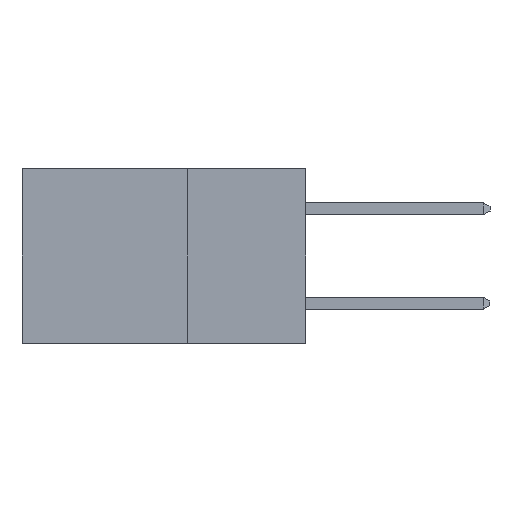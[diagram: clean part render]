
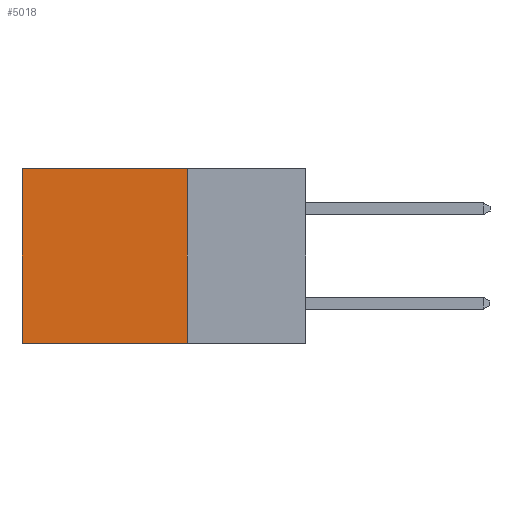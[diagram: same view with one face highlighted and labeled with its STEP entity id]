
A CAD part, left-side view. The second image highlights one B-rep face of the part: STEP entity #5018.
In plain terms, the highlighted planar face has unit normal (-1, 0, 0).
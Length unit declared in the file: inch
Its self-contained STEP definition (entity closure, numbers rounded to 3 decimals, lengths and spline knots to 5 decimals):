
#1595 = CARTESIAN_POINT ( 'NONE',  ( 0.298, 0.25, 0. ) ) ;
#2905 = LINE ( 'NONE', #28155, #13334 ) ;
#3591 = DIRECTION ( 'NONE',  ( 0., 0., -1. ) ) ;
#3656 = DIRECTION ( 'NONE',  ( 1., 0., 0. ) ) ;
#3760 = CARTESIAN_POINT ( 'NONE',  ( 0.298, 0.25, 0. ) ) ;
#3826 = CARTESIAN_POINT ( 'NONE',  ( 0.298, 0.25, -0.37 ) ) ;
#3869 = PLANE ( 'NONE',  #18601 ) ;
#3949 = VERTEX_POINT ( 'NONE', #1595 ) ;
#4423 = CARTESIAN_POINT ( 'NONE',  ( 0.298, 0.25, 0. ) ) ;
#4976 = ORIENTED_EDGE ( 'NONE', *, *, #10635, .T. ) ;
#5018 = ADVANCED_FACE ( 'NONE', ( #29921 ), #3869, .F. ) ;
#6006 = LINE ( 'NONE', #4423, #11601 ) ;
#8602 = VERTEX_POINT ( 'NONE', #27723 ) ;
#9657 = ORIENTED_EDGE ( 'NONE', *, *, #11006, .F. ) ;
#10635 = EDGE_CURVE ( 'NONE', #8602, #29843, #15673, .T. ) ;
#10857 = LINE ( 'NONE', #3826, #23388 ) ;
#11006 = EDGE_CURVE ( 'NONE', #3949, #22201, #6006, .T. ) ;
#11049 = ORIENTED_EDGE ( 'NONE', *, *, #20046, .F. ) ;
#11155 = DIRECTION ( 'NONE',  ( 0., 0., -1. ) ) ;
#11582 = EDGE_LOOP ( 'NONE', ( #4976, #11049, #9657, #17369 ) ) ;
#11601 = VECTOR ( 'NONE', #23367, 39.37008 ) ;
#13334 = VECTOR ( 'NONE', #16445, 39.37008 ) ;
#15673 = LINE ( 'NONE', #15886, #21914 ) ;
#15886 = CARTESIAN_POINT ( 'NONE',  ( 0.298, 0.6, 0. ) ) ;
#16445 = DIRECTION ( 'NONE',  ( 0., 1., 0. ) ) ;
#17369 = ORIENTED_EDGE ( 'NONE', *, *, #21478, .T. ) ;
#18601 = AXIS2_PLACEMENT_3D ( 'NONE', #3760, #3656, #3591 ) ;
#20046 = EDGE_CURVE ( 'NONE', #22201, #29843, #10857, .T. ) ;
#20368 = DIRECTION ( 'NONE',  ( 0., 1., 0. ) ) ;
#21215 = CARTESIAN_POINT ( 'NONE',  ( 0.298, 0.25, -0.37 ) ) ;
#21478 = EDGE_CURVE ( 'NONE', #3949, #8602, #2905, .T. ) ;
#21914 = VECTOR ( 'NONE', #11155, 39.37008 ) ;
#22201 = VERTEX_POINT ( 'NONE', #21215 ) ;
#23367 = DIRECTION ( 'NONE',  ( 0., 0., -1. ) ) ;
#23388 = VECTOR ( 'NONE', #20368, 39.37008 ) ;
#24384 = CARTESIAN_POINT ( 'NONE',  ( 0.298, 0.6, -0.37 ) ) ;
#27723 = CARTESIAN_POINT ( 'NONE',  ( 0.298, 0.6, 0. ) ) ;
#28155 = CARTESIAN_POINT ( 'NONE',  ( 0.298, 0.25, 0. ) ) ;
#29843 = VERTEX_POINT ( 'NONE', #24384 ) ;
#29921 = FACE_OUTER_BOUND ( 'NONE', #11582, .T. ) ;
